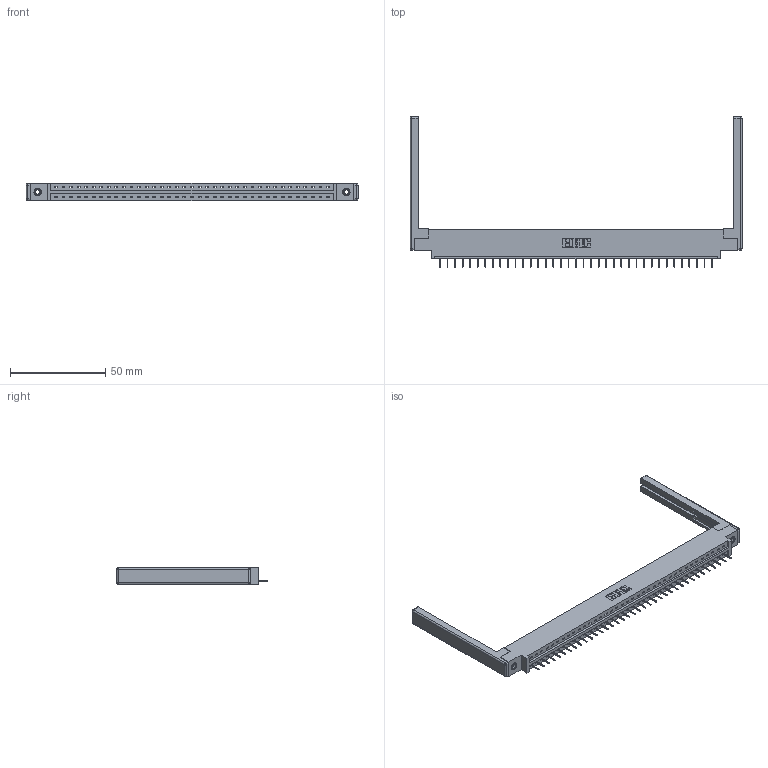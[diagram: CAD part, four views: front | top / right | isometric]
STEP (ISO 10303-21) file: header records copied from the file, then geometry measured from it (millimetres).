
FILE_DESCRIPTION (( 'STEP AP203' ), '1' );
FILE_NAME ('387-037-524-668.STEP', '2019-10-04T14:34:14', ( '' ), ( '' ), 'SwSTEP 2.0', 'SolidWorks 2016', '' );
FILE_SCHEMA (( 'CONFIG_CONTROL_DESIGN' ));
Length unit declared in the file: inch
Products named in the file (5): 345-250-001_345-250-001-102; 307-220-068; 387-037-524-668; 337 Part_0.170 Offset - 0.156 Dia-TI; 345-292-001_345-293-124
Assembly tree (42 placements, depth 2):
  387-037-524-668
    337 Part_0.170 Offset - 0.156 Dia-TI
    345-292-001_345-293-124  x37
    345-250-001_345-250-001-102  x2
    307-220-068  x2
Bounding box: 174.04 x 78.75 x 9.4 mm (x, y, z)
Volume: 22153.6 mm3; surface area: 22002.2 mm2
Topology: 42 solids, 42 shells, 2714 faces, 7817 edges, 5042 vertices
Faces by surface type: plane 2086, cylinder 604, cone 12, sphere 8, torus 4
Entity records: 31116 total; most frequent: CARTESIAN_POINT 5374, ORIENTED_EDGE 5336, DIRECTION 4608, EDGE_CURVE 2668, VECTOR 2494, LINE 2494, VERTEX_POINT 1766, AXIS2_PLACEMENT_3D 1057
